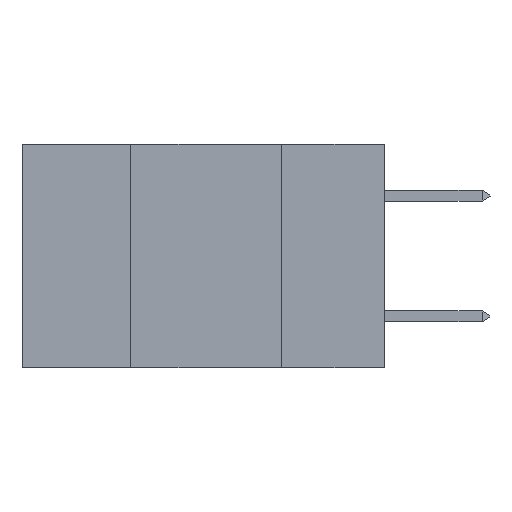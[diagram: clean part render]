
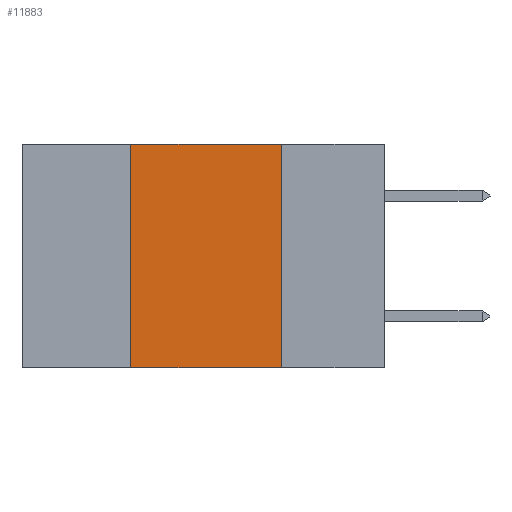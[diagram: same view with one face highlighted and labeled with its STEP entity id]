
A CAD part, left-side view. The second image highlights one B-rep face of the part: STEP entity #11883.
In plain terms, the highlighted planar face has unit normal (-1, 0, 0).
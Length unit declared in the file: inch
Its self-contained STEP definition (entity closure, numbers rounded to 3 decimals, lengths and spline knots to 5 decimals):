
#757 = PLANE ( 'NONE',  #9701 ) ;
#1342 = EDGE_CURVE ( 'NONE', #9148, #7263, #6648, .T. ) ;
#2106 = CARTESIAN_POINT ( 'NONE',  ( 0., 0.42, 0. ) ) ;
#2719 = FACE_OUTER_BOUND ( 'NONE', #5745, .T. ) ;
#2894 = ORIENTED_EDGE ( 'NONE', *, *, #7618, .T. ) ;
#3325 = CARTESIAN_POINT ( 'NONE',  ( 0., 0.17, 0. ) ) ;
#3865 = CARTESIAN_POINT ( 'NONE',  ( 0., 0.17, 0. ) ) ;
#4594 = CARTESIAN_POINT ( 'NONE',  ( 0., 0.6, 0. ) ) ;
#4677 = CARTESIAN_POINT ( 'NONE',  ( 0., 0.6, 0. ) ) ;
#4901 = VECTOR ( 'NONE', #10431, 39.37008 ) ;
#4971 = VERTEX_POINT ( 'NONE', #11172 ) ;
#5022 = CARTESIAN_POINT ( 'NONE',  ( 0., 0.17, -0.37 ) ) ;
#5030 = VECTOR ( 'NONE', #5450, 39.37008 ) ;
#5264 = ORIENTED_EDGE ( 'NONE', *, *, #7110, .F. ) ;
#5450 = DIRECTION ( 'NONE',  ( 0., -1., 0. ) ) ;
#5514 = LINE ( 'NONE', #4594, #5030 ) ;
#5530 = DIRECTION ( 'NONE',  ( 1., 0., 0. ) ) ;
#5745 = EDGE_LOOP ( 'NONE', ( #8535, #5264, #6839, #2894 ) ) ;
#6240 = CARTESIAN_POINT ( 'NONE',  ( 0., 0.42, 0. ) ) ;
#6371 = LINE ( 'NONE', #11073, #7988 ) ;
#6648 = LINE ( 'NONE', #3865, #4901 ) ;
#6839 = ORIENTED_EDGE ( 'NONE', *, *, #9051, .F. ) ;
#7110 = EDGE_CURVE ( 'NONE', #9587, #9148, #5514, .T. ) ;
#7263 = VERTEX_POINT ( 'NONE', #5022 ) ;
#7299 = VECTOR ( 'NONE', #9555, 39.37008 ) ;
#7618 = EDGE_CURVE ( 'NONE', #4971, #7263, #6371, .T. ) ;
#7988 = VECTOR ( 'NONE', #9398, 39.37008 ) ;
#8535 = ORIENTED_EDGE ( 'NONE', *, *, #1342, .F. ) ;
#9051 = EDGE_CURVE ( 'NONE', #4971, #9587, #10490, .T. ) ;
#9111 = DIRECTION ( 'NONE',  ( 0., 0., -1. ) ) ;
#9148 = VERTEX_POINT ( 'NONE', #3325 ) ;
#9398 = DIRECTION ( 'NONE',  ( 0., -1., 0. ) ) ;
#9555 = DIRECTION ( 'NONE',  ( 0., 0., 1. ) ) ;
#9587 = VERTEX_POINT ( 'NONE', #6240 ) ;
#9701 = AXIS2_PLACEMENT_3D ( 'NONE', #4677, #5530, #9111 ) ;
#10431 = DIRECTION ( 'NONE',  ( 0., 0., -1. ) ) ;
#10490 = LINE ( 'NONE', #2106, #7299 ) ;
#11073 = CARTESIAN_POINT ( 'NONE',  ( 0., 0.6, -0.37 ) ) ;
#11172 = CARTESIAN_POINT ( 'NONE',  ( 0., 0.42, -0.37 ) ) ;
#11883 = ADVANCED_FACE ( 'NONE', ( #2719 ), #757, .F. ) ;
